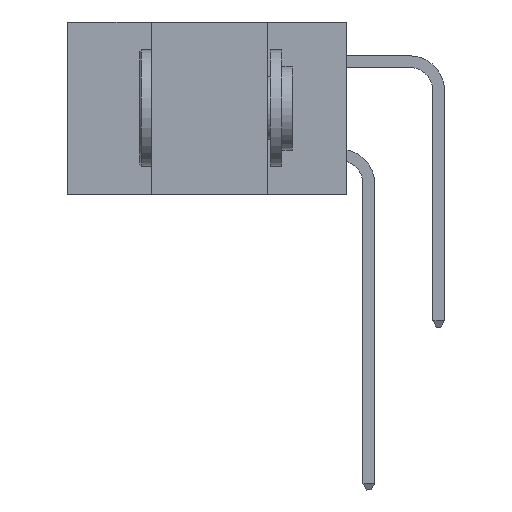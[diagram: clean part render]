
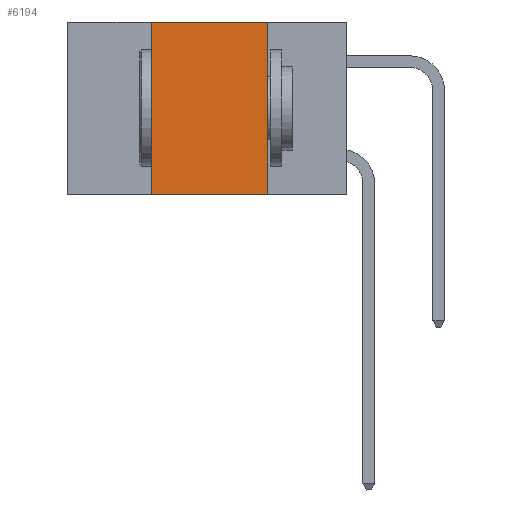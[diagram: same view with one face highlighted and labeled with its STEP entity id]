
A CAD part, left-side view. The second image highlights one B-rep face of the part: STEP entity #6194.
In plain terms, the highlighted planar face has unit normal (-1, 0, 0).
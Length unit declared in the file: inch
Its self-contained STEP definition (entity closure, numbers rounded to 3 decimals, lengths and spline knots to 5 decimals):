
#60 = VECTOR ( 'NONE', #11915, 39.37008 ) ;
#299 = VECTOR ( 'NONE', #14050, 39.37008 ) ;
#336 = DIRECTION ( 'NONE',  ( 1., 0., 0. ) ) ;
#2389 = CARTESIAN_POINT ( 'NONE',  ( 0., 0.6, -0.37 ) ) ;
#2454 = CARTESIAN_POINT ( 'NONE',  ( 0., 0.17, 0. ) ) ;
#2665 = VERTEX_POINT ( 'NONE', #19561 ) ;
#3410 = CARTESIAN_POINT ( 'NONE',  ( 0., 0.17, 0. ) ) ;
#5183 = LINE ( 'NONE', #21419, #60 ) ;
#5568 = LINE ( 'NONE', #14935, #20328 ) ;
#5691 = FACE_OUTER_BOUND ( 'NONE', #8095, .T. ) ;
#6194 = ADVANCED_FACE ( 'NONE', ( #5691 ), #11961, .F. ) ;
#7935 = ORIENTED_EDGE ( 'NONE', *, *, #22933, .F. ) ;
#8095 = EDGE_LOOP ( 'NONE', ( #7935, #10936, #11837, #23177 ) ) ;
#8357 = VERTEX_POINT ( 'NONE', #11017 ) ;
#10936 = ORIENTED_EDGE ( 'NONE', *, *, #16581, .F. ) ;
#11017 = CARTESIAN_POINT ( 'NONE',  ( 0., 0.42, 0. ) ) ;
#11837 = ORIENTED_EDGE ( 'NONE', *, *, #22187, .F. ) ;
#11915 = DIRECTION ( 'NONE',  ( 0., -1., 0. ) ) ;
#11961 = PLANE ( 'NONE',  #14366 ) ;
#12035 = EDGE_CURVE ( 'NONE', #14544, #2665, #20185, .T. ) ;
#13918 = DIRECTION ( 'NONE',  ( 0., 0., -1. ) ) ;
#14050 = DIRECTION ( 'NONE',  ( 0., -1., 0. ) ) ;
#14366 = AXIS2_PLACEMENT_3D ( 'NONE', #21467, #336, #13918 ) ;
#14544 = VERTEX_POINT ( 'NONE', #20676 ) ;
#14935 = CARTESIAN_POINT ( 'NONE',  ( 0., 0.42, 0. ) ) ;
#16581 = EDGE_CURVE ( 'NONE', #8357, #21860, #5183, .T. ) ;
#16856 = DIRECTION ( 'NONE',  ( 0., 0., 1. ) ) ;
#17080 = DIRECTION ( 'NONE',  ( 0., 0., -1. ) ) ;
#18227 = VECTOR ( 'NONE', #17080, 39.37008 ) ;
#19561 = CARTESIAN_POINT ( 'NONE',  ( 0., 0.17, -0.37 ) ) ;
#20185 = LINE ( 'NONE', #2389, #299 ) ;
#20328 = VECTOR ( 'NONE', #16856, 39.37008 ) ;
#20676 = CARTESIAN_POINT ( 'NONE',  ( 0., 0.42, -0.37 ) ) ;
#21419 = CARTESIAN_POINT ( 'NONE',  ( 0., 0.6, 0. ) ) ;
#21467 = CARTESIAN_POINT ( 'NONE',  ( 0., 0.6, 0. ) ) ;
#21860 = VERTEX_POINT ( 'NONE', #2454 ) ;
#22187 = EDGE_CURVE ( 'NONE', #14544, #8357, #5568, .T. ) ;
#22933 = EDGE_CURVE ( 'NONE', #21860, #2665, #23253, .T. ) ;
#23177 = ORIENTED_EDGE ( 'NONE', *, *, #12035, .T. ) ;
#23253 = LINE ( 'NONE', #3410, #18227 ) ;
